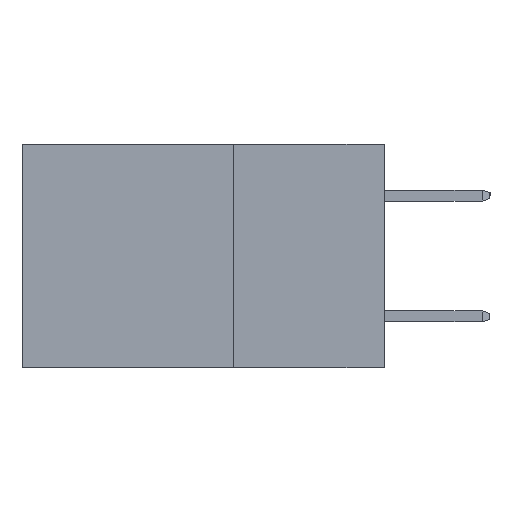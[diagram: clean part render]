
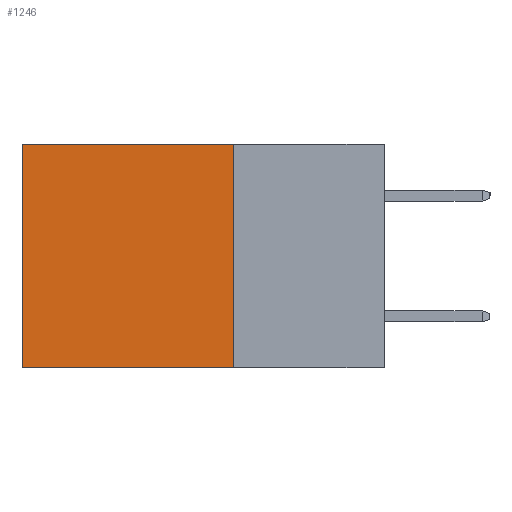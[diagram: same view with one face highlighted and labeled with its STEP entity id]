
A CAD part, left-side view. The second image highlights one B-rep face of the part: STEP entity #1246.
In plain terms, the highlighted planar face has unit normal (-1, 0, 0).
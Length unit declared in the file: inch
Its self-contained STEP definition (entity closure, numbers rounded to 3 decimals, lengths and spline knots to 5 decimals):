
#198 = VECTOR ( 'NONE', #8595, 39.37008 ) ;
#1246 = ADVANCED_FACE ( 'NONE', ( #1842 ), #18710, .F. ) ;
#1842 = FACE_OUTER_BOUND ( 'NONE', #20715, .T. ) ;
#1897 = EDGE_CURVE ( 'NONE', #20025, #16150, #6243, .T. ) ;
#1900 = EDGE_CURVE ( 'NONE', #3573, #16150, #17877, .T. ) ;
#2859 = DIRECTION ( 'NONE',  ( 0., 1., 0. ) ) ;
#3573 = VERTEX_POINT ( 'NONE', #13793 ) ;
#4367 = VECTOR ( 'NONE', #19238, 39.37008 ) ;
#5428 = LINE ( 'NONE', #12145, #4367 ) ;
#6243 = LINE ( 'NONE', #11199, #20398 ) ;
#6401 = EDGE_CURVE ( 'NONE', #14197, #20025, #5428, .T. ) ;
#6596 = EDGE_CURVE ( 'NONE', #14197, #3573, #11907, .T. ) ;
#7300 = ORIENTED_EDGE ( 'NONE', *, *, #1900, .F. ) ;
#8065 = ORIENTED_EDGE ( 'NONE', *, *, #1897, .T. ) ;
#8595 = DIRECTION ( 'NONE',  ( 0., 0., -1. ) ) ;
#10277 = DIRECTION ( 'NONE',  ( 1., 0., 0. ) ) ;
#11199 = CARTESIAN_POINT ( 'NONE',  ( 0.2615, 0.6, -0.37 ) ) ;
#11907 = LINE ( 'NONE', #15088, #198 ) ;
#12145 = CARTESIAN_POINT ( 'NONE',  ( 0.2615, 0.25, 0. ) ) ;
#12757 = DIRECTION ( 'NONE',  ( 0., 0., -1. ) ) ;
#13793 = CARTESIAN_POINT ( 'NONE',  ( 0.2615, 0.25, -0.37 ) ) ;
#14153 = CARTESIAN_POINT ( 'NONE',  ( 0.2615, 0.6, 0. ) ) ;
#14197 = VERTEX_POINT ( 'NONE', #20211 ) ;
#14406 = CARTESIAN_POINT ( 'NONE',  ( 0.2615, 0.25, -0.37 ) ) ;
#14603 = ORIENTED_EDGE ( 'NONE', *, *, #6596, .F. ) ;
#15088 = CARTESIAN_POINT ( 'NONE',  ( 0.2615, 0.25, -0.37 ) ) ;
#16150 = VERTEX_POINT ( 'NONE', #18353 ) ;
#16589 = VECTOR ( 'NONE', #2859, 39.37008 ) ;
#17877 = LINE ( 'NONE', #14406, #16589 ) ;
#18353 = CARTESIAN_POINT ( 'NONE',  ( 0.2615, 0.6, -0.37 ) ) ;
#18673 = ORIENTED_EDGE ( 'NONE', *, *, #6401, .T. ) ;
#18710 = PLANE ( 'NONE',  #19354 ) ;
#19238 = DIRECTION ( 'NONE',  ( 0., 1., 0. ) ) ;
#19354 = AXIS2_PLACEMENT_3D ( 'NONE', #20159, #10277, #20354 ) ;
#20025 = VERTEX_POINT ( 'NONE', #14153 ) ;
#20159 = CARTESIAN_POINT ( 'NONE',  ( 0.2615, 0.25, -0.37 ) ) ;
#20211 = CARTESIAN_POINT ( 'NONE',  ( 0.2615, 0.25, 0. ) ) ;
#20354 = DIRECTION ( 'NONE',  ( 0., 0., -1. ) ) ;
#20398 = VECTOR ( 'NONE', #12757, 39.37008 ) ;
#20715 = EDGE_LOOP ( 'NONE', ( #8065, #7300, #14603, #18673 ) ) ;
